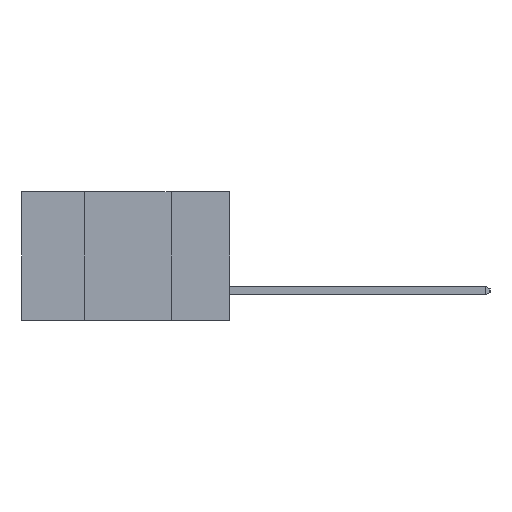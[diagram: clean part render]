
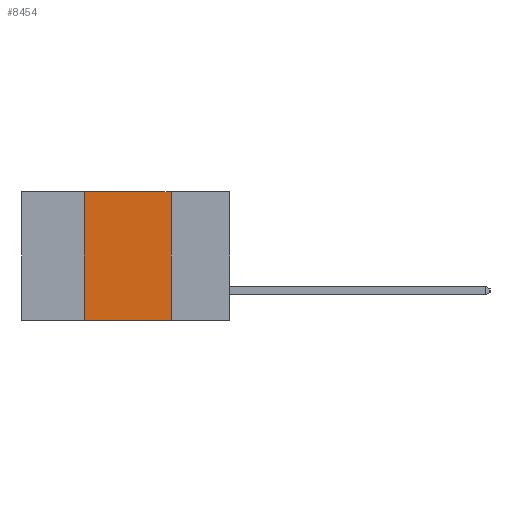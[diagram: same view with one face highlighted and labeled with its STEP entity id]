
A CAD part, left-side view. The second image highlights one B-rep face of the part: STEP entity #8454.
In plain terms, the highlighted planar face has unit normal (-1, 0, 0).
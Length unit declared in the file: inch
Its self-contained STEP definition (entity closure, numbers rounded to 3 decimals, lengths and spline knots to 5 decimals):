
#130 = VECTOR ( 'NONE', #16943, 39.37008 ) ;
#285 = CARTESIAN_POINT ( 'NONE',  ( 0., 0.17, 0. ) ) ;
#712 = VERTEX_POINT ( 'NONE', #13606 ) ;
#1582 = ORIENTED_EDGE ( 'NONE', *, *, #14682, .F. ) ;
#1788 = VECTOR ( 'NONE', #15285, 39.37008 ) ;
#1899 = PLANE ( 'NONE',  #13413 ) ;
#1968 = DIRECTION ( 'NONE',  ( 1., 0., 0. ) ) ;
#2086 = ORIENTED_EDGE ( 'NONE', *, *, #15691, .F. ) ;
#2562 = ORIENTED_EDGE ( 'NONE', *, *, #17637, .T. ) ;
#3165 = CARTESIAN_POINT ( 'NONE',  ( 0., 0.6, 0. ) ) ;
#4752 = VERTEX_POINT ( 'NONE', #6507 ) ;
#4864 = LINE ( 'NONE', #3165, #130 ) ;
#6507 = CARTESIAN_POINT ( 'NONE',  ( 0., 0.42, 0. ) ) ;
#6584 = CARTESIAN_POINT ( 'NONE',  ( 0., 0.42, -0.37 ) ) ;
#7060 = VECTOR ( 'NONE', #12794, 39.37008 ) ;
#7538 = LINE ( 'NONE', #285, #7060 ) ;
#8454 = ADVANCED_FACE ( 'NONE', ( #11958 ), #1899, .F. ) ;
#8687 = VECTOR ( 'NONE', #16713, 39.37008 ) ;
#9203 = VERTEX_POINT ( 'NONE', #14714 ) ;
#9856 = ORIENTED_EDGE ( 'NONE', *, *, #18329, .F. ) ;
#10640 = CARTESIAN_POINT ( 'NONE',  ( 0., 0.42, 0. ) ) ;
#10878 = VERTEX_POINT ( 'NONE', #6584 ) ;
#11276 = CARTESIAN_POINT ( 'NONE',  ( 0., 0.6, 0. ) ) ;
#11958 = FACE_OUTER_BOUND ( 'NONE', #16937, .T. ) ;
#12794 = DIRECTION ( 'NONE',  ( 0., 0., -1. ) ) ;
#12839 = DIRECTION ( 'NONE',  ( 0., 0., -1. ) ) ;
#13413 = AXIS2_PLACEMENT_3D ( 'NONE', #11276, #1968, #12839 ) ;
#13606 = CARTESIAN_POINT ( 'NONE',  ( 0., 0.17, 0. ) ) ;
#14682 = EDGE_CURVE ( 'NONE', #712, #9203, #7538, .T. ) ;
#14714 = CARTESIAN_POINT ( 'NONE',  ( 0., 0.17, -0.37 ) ) ;
#15285 = DIRECTION ( 'NONE',  ( 0., -1., 0. ) ) ;
#15691 = EDGE_CURVE ( 'NONE', #10878, #4752, #16763, .T. ) ;
#16713 = DIRECTION ( 'NONE',  ( 0., 0., 1. ) ) ;
#16763 = LINE ( 'NONE', #10640, #8687 ) ;
#16937 = EDGE_LOOP ( 'NONE', ( #1582, #9856, #2086, #2562 ) ) ;
#16943 = DIRECTION ( 'NONE',  ( 0., -1., 0. ) ) ;
#17637 = EDGE_CURVE ( 'NONE', #10878, #9203, #18469, .T. ) ;
#18329 = EDGE_CURVE ( 'NONE', #4752, #712, #4864, .T. ) ;
#18469 = LINE ( 'NONE', #19517, #1788 ) ;
#19517 = CARTESIAN_POINT ( 'NONE',  ( 0., 0.6, -0.37 ) ) ;
